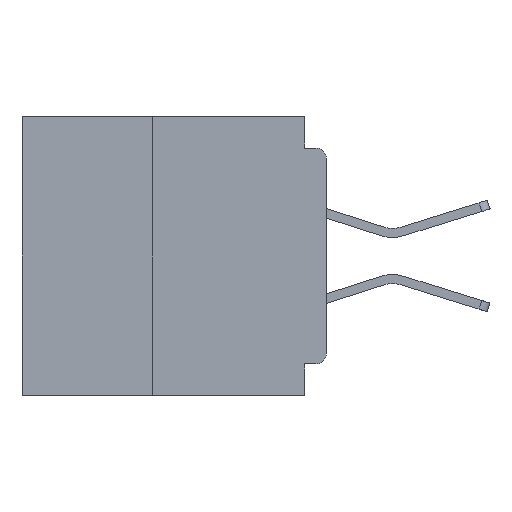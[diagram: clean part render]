
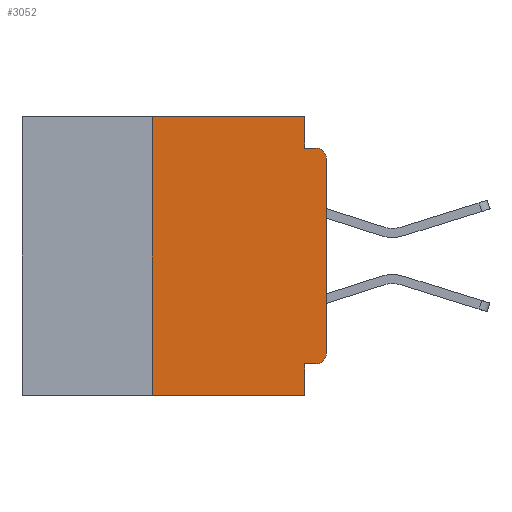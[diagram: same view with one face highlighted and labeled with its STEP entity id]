
A CAD part, left-side view. The second image highlights one B-rep face of the part: STEP entity #3052.
In plain terms, the highlighted planar face has unit normal (-1, 0, 0).
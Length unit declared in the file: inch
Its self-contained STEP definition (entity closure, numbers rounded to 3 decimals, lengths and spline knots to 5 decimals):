
#145 = LINE ( 'NONE', #1793, #32595 ) ;
#394 = EDGE_CURVE ( 'NONE', #14068, #22326, #36413, .T. ) ;
#1311 = CARTESIAN_POINT ( 'NONE',  ( 0., 0.437, 0. ) ) ;
#1417 = ORIENTED_EDGE ( 'NONE', *, *, #394, .F. ) ;
#1793 = CARTESIAN_POINT ( 'NONE',  ( 0., 0., 0. ) ) ;
#1811 = VECTOR ( 'NONE', #39572, 39.37008 ) ;
#3052 = ADVANCED_FACE ( 'NONE', ( #16255 ), #31585, .F. ) ;
#3240 = VECTOR ( 'NONE', #10405, 39.37008 ) ;
#3334 = DIRECTION ( 'NONE',  ( 0., 0., 1. ) ) ;
#3602 = DIRECTION ( 'NONE',  ( 1., 0., 0. ) ) ;
#3772 = VERTEX_POINT ( 'NONE', #22372 ) ;
#3849 = VERTEX_POINT ( 'NONE', #16545 ) ;
#4401 = VERTEX_POINT ( 'NONE', #13640 ) ;
#4992 = DIRECTION ( 'NONE',  ( 0., 0., 1. ) ) ;
#5136 = AXIS2_PLACEMENT_3D ( 'NONE', #11377, #33193, #14569 ) ;
#7056 = CARTESIAN_POINT ( 'NONE',  ( 0., 0.031, -0.045 ) ) ;
#7788 = LINE ( 'NONE', #10639, #24460 ) ;
#7906 = EDGE_CURVE ( 'NONE', #12112, #14068, #25892, .T. ) ;
#10070 = EDGE_CURVE ( 'NONE', #4401, #22326, #11458, .T. ) ;
#10405 = DIRECTION ( 'NONE',  ( 0., -1., 0. ) ) ;
#10409 = ORIENTED_EDGE ( 'NONE', *, *, #24242, .T. ) ;
#10485 = EDGE_LOOP ( 'NONE', ( #25949, #16792, #1417, #35844, #36987, #38240, #12357, #17219, #40026, #10409 ) ) ;
#10639 = CARTESIAN_POINT ( 'NONE',  ( 0., 0.437, -0.4 ) ) ;
#11377 = CARTESIAN_POINT ( 'NONE',  ( 0., 0.015, -0.34 ) ) ;
#11458 = CIRCLE ( 'NONE', #12494, 0.015 ) ;
#12112 = VERTEX_POINT ( 'NONE', #17932 ) ;
#12247 = LINE ( 'NONE', #21976, #36143 ) ;
#12314 = EDGE_CURVE ( 'NONE', #16417, #34717, #12247, .T. ) ;
#12357 = ORIENTED_EDGE ( 'NONE', *, *, #39419, .T. ) ;
#12494 = AXIS2_PLACEMENT_3D ( 'NONE', #32096, #13428, #35207 ) ;
#12650 = CARTESIAN_POINT ( 'NONE',  ( 0., 0.25, -0.4 ) ) ;
#13105 = DIRECTION ( 'NONE',  ( 0., 0., -1. ) ) ;
#13428 = DIRECTION ( 'NONE',  ( -1., 0., 0. ) ) ;
#13640 = CARTESIAN_POINT ( 'NONE',  ( 0., 0., -0.06 ) ) ;
#14068 = VERTEX_POINT ( 'NONE', #7056 ) ;
#14569 = DIRECTION ( 'NONE',  ( 0., 0., -1. ) ) ;
#15595 = CARTESIAN_POINT ( 'NONE',  ( 0., 0.25, 0. ) ) ;
#15899 = CARTESIAN_POINT ( 'NONE',  ( 0., 0.25, -0.4 ) ) ;
#16255 = FACE_OUTER_BOUND ( 'NONE', #10485, .T. ) ;
#16307 = CIRCLE ( 'NONE', #5136, 0.015 ) ;
#16417 = VERTEX_POINT ( 'NONE', #26457 ) ;
#16545 = CARTESIAN_POINT ( 'NONE',  ( 0., 0., -0.34 ) ) ;
#16792 = ORIENTED_EDGE ( 'NONE', *, *, #10070, .T. ) ;
#17219 = ORIENTED_EDGE ( 'NONE', *, *, #12314, .F. ) ;
#17345 = VECTOR ( 'NONE', #3334, 39.37008 ) ;
#17932 = CARTESIAN_POINT ( 'NONE',  ( 0., 0.031, 0. ) ) ;
#21481 = AXIS2_PLACEMENT_3D ( 'NONE', #1311, #3602, #13105 ) ;
#21976 = CARTESIAN_POINT ( 'NONE',  ( 0., 0.031, -0.4 ) ) ;
#22326 = VERTEX_POINT ( 'NONE', #29537 ) ;
#22372 = CARTESIAN_POINT ( 'NONE',  ( 0., 0.015, -0.355 ) ) ;
#22681 = EDGE_CURVE ( 'NONE', #28606, #28029, #25613, .T. ) ;
#23786 = LINE ( 'NONE', #27967, #39363 ) ;
#23939 = CARTESIAN_POINT ( 'NONE',  ( 0., 0.031, 0. ) ) ;
#24242 = EDGE_CURVE ( 'NONE', #3772, #3849, #16307, .T. ) ;
#24460 = VECTOR ( 'NONE', #34800, 39.37008 ) ;
#24629 = CARTESIAN_POINT ( 'NONE',  ( 0., 0.031, -0.4 ) ) ;
#25613 = LINE ( 'NONE', #15899, #17345 ) ;
#25892 = LINE ( 'NONE', #23939, #1811 ) ;
#25949 = ORIENTED_EDGE ( 'NONE', *, *, #27319, .T. ) ;
#26204 = VECTOR ( 'NONE', #26847, 39.37008 ) ;
#26457 = CARTESIAN_POINT ( 'NONE',  ( 0., 0.031, -0.355 ) ) ;
#26586 = CARTESIAN_POINT ( 'NONE',  ( 0., 0., -0.045 ) ) ;
#26847 = DIRECTION ( 'NONE',  ( 0., -1., 0. ) ) ;
#27319 = EDGE_CURVE ( 'NONE', #3849, #4401, #145, .T. ) ;
#27511 = EDGE_CURVE ( 'NONE', #3772, #16417, #23786, .T. ) ;
#27967 = CARTESIAN_POINT ( 'NONE',  ( 0., 0., -0.355 ) ) ;
#28029 = VERTEX_POINT ( 'NONE', #15595 ) ;
#28114 = DIRECTION ( 'NONE',  ( 0., 0., -1. ) ) ;
#28606 = VERTEX_POINT ( 'NONE', #12650 ) ;
#29537 = CARTESIAN_POINT ( 'NONE',  ( 0., 0.015, -0.045 ) ) ;
#31105 = DIRECTION ( 'NONE',  ( 0., 1., 0. ) ) ;
#31585 = PLANE ( 'NONE',  #21481 ) ;
#31603 = EDGE_CURVE ( 'NONE', #28029, #12112, #37469, .T. ) ;
#32096 = CARTESIAN_POINT ( 'NONE',  ( 0., 0.015, -0.06 ) ) ;
#32261 = CARTESIAN_POINT ( 'NONE',  ( 0., 0.437, 0. ) ) ;
#32595 = VECTOR ( 'NONE', #4992, 39.37008 ) ;
#33193 = DIRECTION ( 'NONE',  ( -1., 0., 0. ) ) ;
#34717 = VERTEX_POINT ( 'NONE', #24629 ) ;
#34800 = DIRECTION ( 'NONE',  ( 0., -1., 0. ) ) ;
#35207 = DIRECTION ( 'NONE',  ( 0., 0., -1. ) ) ;
#35844 = ORIENTED_EDGE ( 'NONE', *, *, #7906, .F. ) ;
#36143 = VECTOR ( 'NONE', #28114, 39.37008 ) ;
#36413 = LINE ( 'NONE', #26586, #26204 ) ;
#36987 = ORIENTED_EDGE ( 'NONE', *, *, #31603, .F. ) ;
#37469 = LINE ( 'NONE', #32261, #3240 ) ;
#38240 = ORIENTED_EDGE ( 'NONE', *, *, #22681, .F. ) ;
#39363 = VECTOR ( 'NONE', #31105, 39.37008 ) ;
#39419 = EDGE_CURVE ( 'NONE', #28606, #34717, #7788, .T. ) ;
#39572 = DIRECTION ( 'NONE',  ( 0., 0., -1. ) ) ;
#40026 = ORIENTED_EDGE ( 'NONE', *, *, #27511, .F. ) ;
